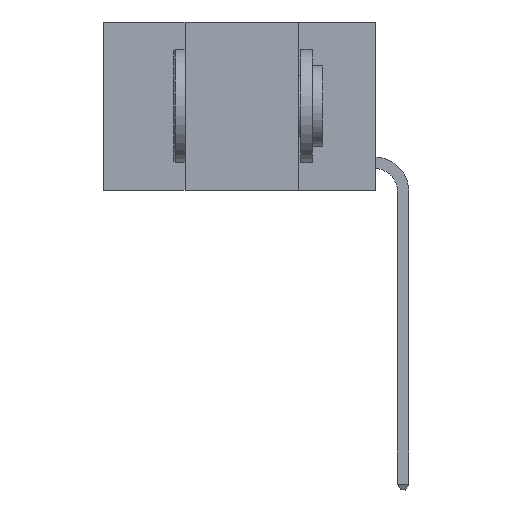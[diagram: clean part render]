
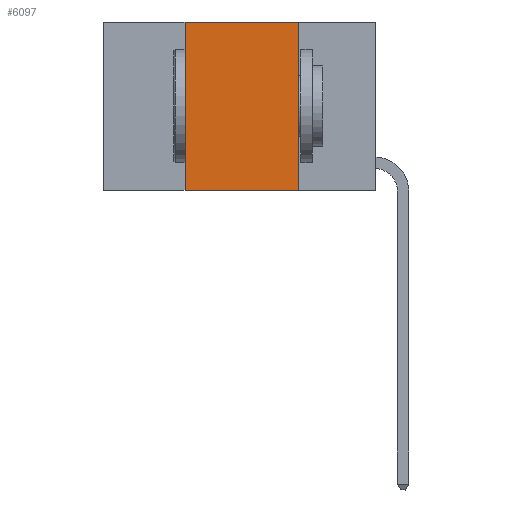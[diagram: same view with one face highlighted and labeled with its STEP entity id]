
A CAD part, left-side view. The second image highlights one B-rep face of the part: STEP entity #6097.
In plain terms, the highlighted planar face has unit normal (-1, 0, 0).
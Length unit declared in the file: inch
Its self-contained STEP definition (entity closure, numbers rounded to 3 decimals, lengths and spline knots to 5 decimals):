
#1959 = EDGE_CURVE ( 'NONE', #3311, #12392, #7191, .T. ) ;
#2388 = LINE ( 'NONE', #17951, #12340 ) ;
#2418 = ORIENTED_EDGE ( 'NONE', *, *, #9593, .F. ) ;
#2457 = DIRECTION ( 'NONE',  ( 0., -1., 0. ) ) ;
#3311 = VERTEX_POINT ( 'NONE', #15164 ) ;
#4369 = DIRECTION ( 'NONE',  ( 0., 0., -1. ) ) ;
#5267 = ORIENTED_EDGE ( 'NONE', *, *, #1959, .F. ) ;
#5717 = ORIENTED_EDGE ( 'NONE', *, *, #7687, .F. ) ;
#5831 = EDGE_CURVE ( 'NONE', #15930, #7596, #2388, .T. ) ;
#6097 = ADVANCED_FACE ( 'NONE', ( #8745 ), #17030, .F. ) ;
#6106 = CARTESIAN_POINT ( 'NONE',  ( 0., 0.42, 0. ) ) ;
#7191 = LINE ( 'NONE', #14413, #14759 ) ;
#7564 = DIRECTION ( 'NONE',  ( 0., 0., 1. ) ) ;
#7572 = VECTOR ( 'NONE', #7564, 39.37008 ) ;
#7596 = VERTEX_POINT ( 'NONE', #11646 ) ;
#7687 = EDGE_CURVE ( 'NONE', #15930, #3311, #10911, .T. ) ;
#7723 = DIRECTION ( 'NONE',  ( 0., 0., -1. ) ) ;
#8745 = FACE_OUTER_BOUND ( 'NONE', #10088, .T. ) ;
#9593 = EDGE_CURVE ( 'NONE', #12392, #7596, #9958, .T. ) ;
#9958 = LINE ( 'NONE', #10543, #12880 ) ;
#10088 = EDGE_LOOP ( 'NONE', ( #2418, #5267, #5717, #16988 ) ) ;
#10543 = CARTESIAN_POINT ( 'NONE',  ( 0., 0.17, 0. ) ) ;
#10911 = LINE ( 'NONE', #6106, #7572 ) ;
#11432 = CARTESIAN_POINT ( 'NONE',  ( 0., 0.6, 0. ) ) ;
#11646 = CARTESIAN_POINT ( 'NONE',  ( 0., 0.17, -0.37 ) ) ;
#12157 = CARTESIAN_POINT ( 'NONE',  ( 0., 0.17, 0. ) ) ;
#12340 = VECTOR ( 'NONE', #2457, 39.37008 ) ;
#12392 = VERTEX_POINT ( 'NONE', #12157 ) ;
#12843 = DIRECTION ( 'NONE',  ( 1., 0., 0. ) ) ;
#12880 = VECTOR ( 'NONE', #7723, 39.37008 ) ;
#14316 = DIRECTION ( 'NONE',  ( 0., -1., 0. ) ) ;
#14413 = CARTESIAN_POINT ( 'NONE',  ( 0., 0.6, 0. ) ) ;
#14759 = VECTOR ( 'NONE', #14316, 39.37008 ) ;
#15164 = CARTESIAN_POINT ( 'NONE',  ( 0., 0.42, 0. ) ) ;
#15374 = AXIS2_PLACEMENT_3D ( 'NONE', #11432, #12843, #4369 ) ;
#15930 = VERTEX_POINT ( 'NONE', #17553 ) ;
#16988 = ORIENTED_EDGE ( 'NONE', *, *, #5831, .T. ) ;
#17030 = PLANE ( 'NONE',  #15374 ) ;
#17553 = CARTESIAN_POINT ( 'NONE',  ( 0., 0.42, -0.37 ) ) ;
#17951 = CARTESIAN_POINT ( 'NONE',  ( 0., 0.6, -0.37 ) ) ;
